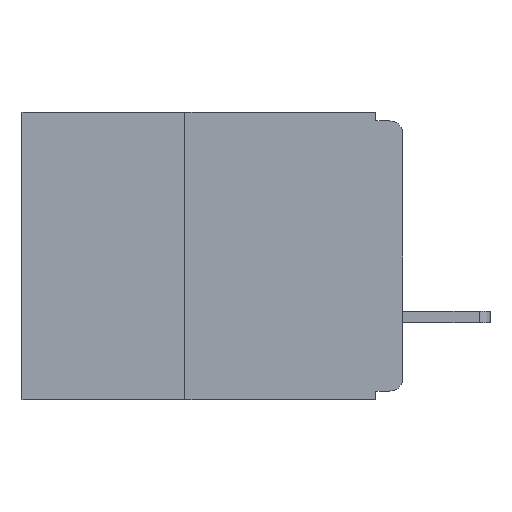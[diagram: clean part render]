
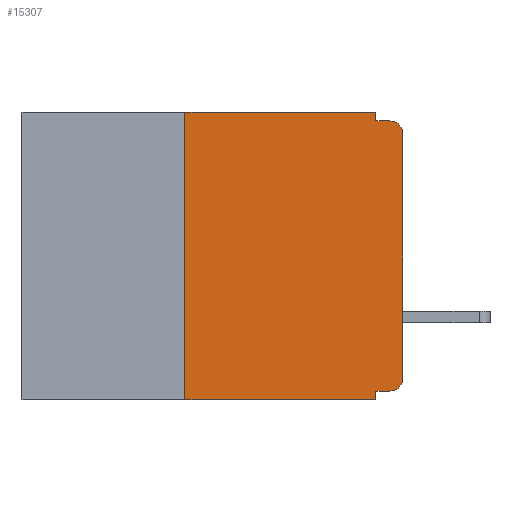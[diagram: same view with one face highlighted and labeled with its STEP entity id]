
A CAD part, left-side view. The second image highlights one B-rep face of the part: STEP entity #15307.
In plain terms, the highlighted planar face has unit normal (-1, 0, 0).
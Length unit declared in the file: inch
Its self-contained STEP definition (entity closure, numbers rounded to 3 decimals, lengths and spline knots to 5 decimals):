
#422 = VERTEX_POINT ( 'NONE', #9837 ) ;
#484 = VECTOR ( 'NONE', #8373, 39.37008 ) ;
#680 = VECTOR ( 'NONE', #14262, 39.37008 ) ;
#1513 = VECTOR ( 'NONE', #9769, 39.37008 ) ;
#1642 = DIRECTION ( 'NONE',  ( 0., -1., 0. ) ) ;
#1948 = EDGE_CURVE ( 'NONE', #17528, #22302, #9521, .T. ) ;
#2006 = VERTEX_POINT ( 'NONE', #10379 ) ;
#2056 = CARTESIAN_POINT ( 'NONE',  ( 0., 0.031, -0.33 ) ) ;
#2291 = CARTESIAN_POINT ( 'NONE',  ( 0., 0., 0. ) ) ;
#2583 = DIRECTION ( 'NONE',  ( -1., 0., 0. ) ) ;
#2767 = ORIENTED_EDGE ( 'NONE', *, *, #5062, .T. ) ;
#3459 = LINE ( 'NONE', #20432, #484 ) ;
#3663 = AXIS2_PLACEMENT_3D ( 'NONE', #13040, #2583, #14793 ) ;
#3832 = DIRECTION ( 'NONE',  ( 0., -1., 0. ) ) ;
#4498 = ORIENTED_EDGE ( 'NONE', *, *, #14859, .T. ) ;
#4591 = CARTESIAN_POINT ( 'NONE',  ( 0., 0., -0.025 ) ) ;
#4746 = LINE ( 'NONE', #2056, #680 ) ;
#4770 = CIRCLE ( 'NONE', #7972, 0.015 ) ;
#5062 = EDGE_CURVE ( 'NONE', #18298, #15270, #12321, .T. ) ;
#5239 = ORIENTED_EDGE ( 'NONE', *, *, #18601, .F. ) ;
#5378 = EDGE_LOOP ( 'NONE', ( #14595, #2767, #5239, #18449, #10561, #21949, #16418, #19644, #7245, #4498 ) ) ;
#5657 = CARTESIAN_POINT ( 'NONE',  ( 0., 0.437, 0. ) ) ;
#5965 = DIRECTION ( 'NONE',  ( 0., -1., 0. ) ) ;
#6170 = DIRECTION ( 'NONE',  ( -1., 0., 0. ) ) ;
#6210 = VECTOR ( 'NONE', #16248, 39.37008 ) ;
#6261 = CARTESIAN_POINT ( 'NONE',  ( 0., 0.25, -0.33 ) ) ;
#7245 = ORIENTED_EDGE ( 'NONE', *, *, #13254, .F. ) ;
#7606 = AXIS2_PLACEMENT_3D ( 'NONE', #5657, #21234, #10927 ) ;
#7972 = AXIS2_PLACEMENT_3D ( 'NONE', #16587, #6170, #18295 ) ;
#8373 = DIRECTION ( 'NONE',  ( 0., 1., 0. ) ) ;
#8429 = CARTESIAN_POINT ( 'NONE',  ( 0., 0.031, -0.33 ) ) ;
#8476 = CARTESIAN_POINT ( 'NONE',  ( 0., 0.25, -0.33 ) ) ;
#9192 = PLANE ( 'NONE',  #7606 ) ;
#9275 = EDGE_CURVE ( 'NONE', #17917, #17528, #14026, .T. ) ;
#9521 = LINE ( 'NONE', #11974, #18171 ) ;
#9769 = DIRECTION ( 'NONE',  ( 0., 0., 1. ) ) ;
#9837 = CARTESIAN_POINT ( 'NONE',  ( 0., 0.031, -0.32 ) ) ;
#10379 = CARTESIAN_POINT ( 'NONE',  ( 0., 0., -0.305 ) ) ;
#10561 = ORIENTED_EDGE ( 'NONE', *, *, #9275, .F. ) ;
#10842 = LINE ( 'NONE', #2291, #6210 ) ;
#10927 = DIRECTION ( 'NONE',  ( 0., 0., -1. ) ) ;
#11576 = CARTESIAN_POINT ( 'NONE',  ( 0., 0.015, -0.32 ) ) ;
#11580 = VERTEX_POINT ( 'NONE', #8429 ) ;
#11974 = CARTESIAN_POINT ( 'NONE',  ( 0., 0.031, 0. ) ) ;
#12110 = CARTESIAN_POINT ( 'NONE',  ( 0., 0.437, -0.33 ) ) ;
#12289 = LINE ( 'NONE', #12110, #15807 ) ;
#12321 = CIRCLE ( 'NONE', #3663, 0.015 ) ;
#12374 = DIRECTION ( 'NONE',  ( 0., 0., -1. ) ) ;
#13040 = CARTESIAN_POINT ( 'NONE',  ( 0., 0.015, -0.025 ) ) ;
#13254 = EDGE_CURVE ( 'NONE', #21013, #422, #3459, .T. ) ;
#13484 = VECTOR ( 'NONE', #5965, 39.37008 ) ;
#13550 = EDGE_CURVE ( 'NONE', #2006, #18298, #10842, .T. ) ;
#13788 = CARTESIAN_POINT ( 'NONE',  ( 0., 0.031, -0.01 ) ) ;
#14026 = LINE ( 'NONE', #16384, #13484 ) ;
#14262 = DIRECTION ( 'NONE',  ( 0., 0., -1. ) ) ;
#14595 = ORIENTED_EDGE ( 'NONE', *, *, #13550, .T. ) ;
#14793 = DIRECTION ( 'NONE',  ( 0., 0., -1. ) ) ;
#14859 = EDGE_CURVE ( 'NONE', #21013, #2006, #4770, .T. ) ;
#15242 = EDGE_CURVE ( 'NONE', #422, #11580, #4746, .T. ) ;
#15270 = VERTEX_POINT ( 'NONE', #19457 ) ;
#15307 = ADVANCED_FACE ( 'NONE', ( #17022 ), #9192, .F. ) ;
#15426 = LINE ( 'NONE', #6261, #1513 ) ;
#15445 = CARTESIAN_POINT ( 'NONE',  ( 0., 0.031, 0. ) ) ;
#15807 = VECTOR ( 'NONE', #1642, 39.37008 ) ;
#16248 = DIRECTION ( 'NONE',  ( 0., 0., 1. ) ) ;
#16384 = CARTESIAN_POINT ( 'NONE',  ( 0., 0.437, 0. ) ) ;
#16418 = ORIENTED_EDGE ( 'NONE', *, *, #17575, .T. ) ;
#16587 = CARTESIAN_POINT ( 'NONE',  ( 0., 0.015, -0.305 ) ) ;
#17022 = FACE_OUTER_BOUND ( 'NONE', #5378, .T. ) ;
#17105 = CARTESIAN_POINT ( 'NONE',  ( 0., 0.25, 0. ) ) ;
#17528 = VERTEX_POINT ( 'NONE', #15445 ) ;
#17575 = EDGE_CURVE ( 'NONE', #19698, #11580, #12289, .T. ) ;
#17917 = VERTEX_POINT ( 'NONE', #17105 ) ;
#18171 = VECTOR ( 'NONE', #12374, 39.37008 ) ;
#18295 = DIRECTION ( 'NONE',  ( 0., 0., -1. ) ) ;
#18298 = VERTEX_POINT ( 'NONE', #4591 ) ;
#18449 = ORIENTED_EDGE ( 'NONE', *, *, #1948, .F. ) ;
#18601 = EDGE_CURVE ( 'NONE', #22302, #15270, #21121, .T. ) ;
#19457 = CARTESIAN_POINT ( 'NONE',  ( 0., 0.015, -0.01 ) ) ;
#19644 = ORIENTED_EDGE ( 'NONE', *, *, #15242, .F. ) ;
#19698 = VERTEX_POINT ( 'NONE', #8476 ) ;
#20432 = CARTESIAN_POINT ( 'NONE',  ( 0., 0., -0.32 ) ) ;
#20582 = VECTOR ( 'NONE', #3832, 39.37008 ) ;
#20971 = EDGE_CURVE ( 'NONE', #19698, #17917, #15426, .T. ) ;
#21013 = VERTEX_POINT ( 'NONE', #11576 ) ;
#21121 = LINE ( 'NONE', #21172, #20582 ) ;
#21172 = CARTESIAN_POINT ( 'NONE',  ( 0., 0., -0.01 ) ) ;
#21234 = DIRECTION ( 'NONE',  ( 1., 0., 0. ) ) ;
#21949 = ORIENTED_EDGE ( 'NONE', *, *, #20971, .F. ) ;
#22302 = VERTEX_POINT ( 'NONE', #13788 ) ;
